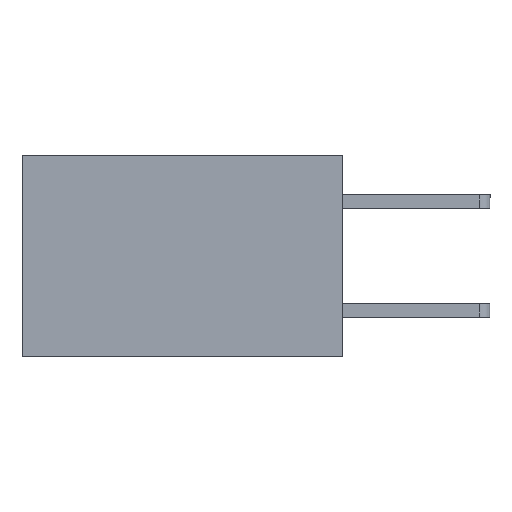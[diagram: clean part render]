
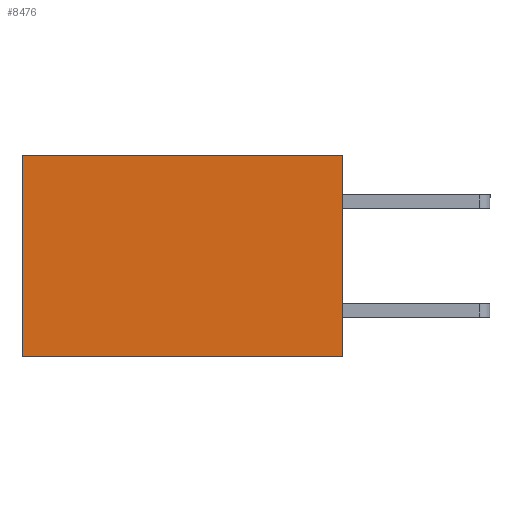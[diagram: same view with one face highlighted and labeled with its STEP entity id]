
A CAD part, left-side view. The second image highlights one B-rep face of the part: STEP entity #8476.
In plain terms, the highlighted planar face has unit normal (-1, 0, 0).
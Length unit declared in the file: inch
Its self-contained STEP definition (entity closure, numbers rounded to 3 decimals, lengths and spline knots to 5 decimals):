
#611 = PLANE ( 'NONE',  #613 ) ;
#613 = AXIS2_PLACEMENT_3D ( 'NONE', #5601, #1363, #6298 ) ;
#1363 = DIRECTION ( 'NONE',  ( 1., 0., 0. ) ) ;
#1463 = LINE ( 'NONE', #8562, #8668 ) ;
#1512 = VERTEX_POINT ( 'NONE', #6517 ) ;
#2057 = CARTESIAN_POINT ( 'NONE',  ( 0.277, 0., -0.37 ) ) ;
#2314 = LINE ( 'NONE', #4744, #7726 ) ;
#2428 = CARTESIAN_POINT ( 'NONE',  ( 0.277, 0.59, -0.37 ) ) ;
#2434 = VECTOR ( 'NONE', #4516, 39.37008 ) ;
#2907 = LINE ( 'NONE', #4525, #8267 ) ;
#3139 = EDGE_CURVE ( 'NONE', #1512, #3791, #2907, .T. ) ;
#3224 = ORIENTED_EDGE ( 'NONE', *, *, #8347, .T. ) ;
#3332 = CARTESIAN_POINT ( 'NONE',  ( 0.277, 0.59, 0. ) ) ;
#3791 = VERTEX_POINT ( 'NONE', #2057 ) ;
#3825 = CARTESIAN_POINT ( 'NONE',  ( 0.277, 0., -0.37 ) ) ;
#4241 = ORIENTED_EDGE ( 'NONE', *, *, #7277, .T. ) ;
#4516 = DIRECTION ( 'NONE',  ( 0., 1., 0. ) ) ;
#4525 = CARTESIAN_POINT ( 'NONE',  ( 0.277, 0., -0.37 ) ) ;
#4553 = DIRECTION ( 'NONE',  ( 0., 0., -1. ) ) ;
#4741 = ORIENTED_EDGE ( 'NONE', *, *, #3139, .F. ) ;
#4744 = CARTESIAN_POINT ( 'NONE',  ( 0.277, 0., 0. ) ) ;
#5163 = EDGE_LOOP ( 'NONE', ( #4241, #7281, #4741, #3224 ) ) ;
#5601 = CARTESIAN_POINT ( 'NONE',  ( 0.277, 0., -0.37 ) ) ;
#5845 = DIRECTION ( 'NONE',  ( 0., 0., -1. ) ) ;
#6122 = VERTEX_POINT ( 'NONE', #2428 ) ;
#6216 = LINE ( 'NONE', #3825, #2434 ) ;
#6298 = DIRECTION ( 'NONE',  ( 0., 0., -1. ) ) ;
#6517 = CARTESIAN_POINT ( 'NONE',  ( 0.277, 0., 0. ) ) ;
#6875 = DIRECTION ( 'NONE',  ( 0., 1., 0. ) ) ;
#7277 = EDGE_CURVE ( 'NONE', #7652, #6122, #1463, .T. ) ;
#7281 = ORIENTED_EDGE ( 'NONE', *, *, #7381, .F. ) ;
#7381 = EDGE_CURVE ( 'NONE', #3791, #6122, #6216, .T. ) ;
#7652 = VERTEX_POINT ( 'NONE', #3332 ) ;
#7726 = VECTOR ( 'NONE', #6875, 39.37008 ) ;
#8267 = VECTOR ( 'NONE', #4553, 39.37008 ) ;
#8347 = EDGE_CURVE ( 'NONE', #1512, #7652, #2314, .T. ) ;
#8476 = ADVANCED_FACE ( 'NONE', ( #8663 ), #611, .F. ) ;
#8562 = CARTESIAN_POINT ( 'NONE',  ( 0.277, 0.59, -0.37 ) ) ;
#8663 = FACE_OUTER_BOUND ( 'NONE', #5163, .T. ) ;
#8668 = VECTOR ( 'NONE', #5845, 39.37008 ) ;
